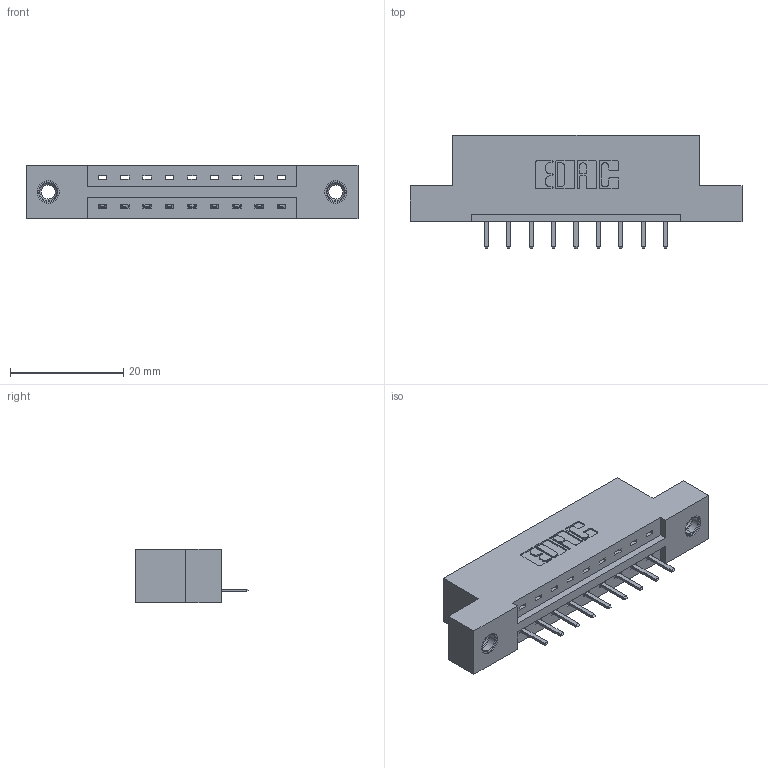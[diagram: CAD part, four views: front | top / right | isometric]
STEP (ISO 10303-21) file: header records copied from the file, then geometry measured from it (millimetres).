
FILE_DESCRIPTION (( 'STEP AP203' ), '1' );
FILE_NAME ('337-009-520-107.STEP', '2019-09-27T19:42:31', ( '' ), ( '' ), 'SwSTEP 2.0', 'SolidWorks 2016', '' );
FILE_SCHEMA (( 'CONFIG_CONTROL_DESIGN' ));
Length unit declared in the file: inch
Products named in the file (4): 345-250-001_345-250-005-103; 345-292-001_345-293-120; 337 Part_Flush Mounting Lugs - 0.156 Dia-TI; 337-009-520-107
Assembly tree (12 placements, depth 2):
  337-009-520-107
    337 Part_Flush Mounting Lugs - 0.156 Dia-TI
    345-292-001_345-293-120  x9
    345-250-001_345-250-005-103  x2
Bounding box: 58.67 x 20.02 x 9.4 mm (x, y, z)
Volume: 5645.8 mm3; surface area: 5598.8 mm2
Topology: 12 solids, 12 shells, 768 faces, 2211 edges, 1442 vertices
Faces by surface type: plane 534, cylinder 218, cone 12, torus 4
Entity records: 12258 total; most frequent: CARTESIAN_POINT 2124, ORIENTED_EDGE 2050, DIRECTION 1877, EDGE_CURVE 1025, VECTOR 873, LINE 873, VERTEX_POINT 676, AXIS2_PLACEMENT_3D 502
